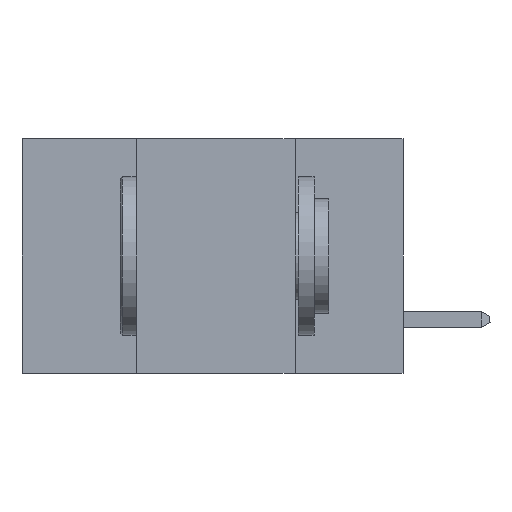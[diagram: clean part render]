
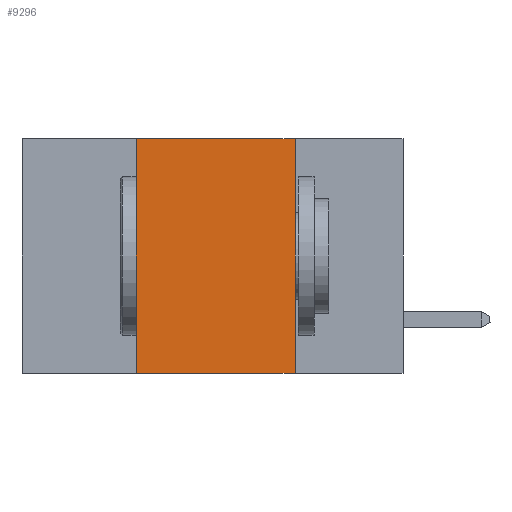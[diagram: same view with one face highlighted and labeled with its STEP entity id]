
A CAD part, left-side view. The second image highlights one B-rep face of the part: STEP entity #9296.
In plain terms, the highlighted planar face has unit normal (-1, 0, 0).
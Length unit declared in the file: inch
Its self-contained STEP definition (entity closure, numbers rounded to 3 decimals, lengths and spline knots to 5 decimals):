
#333 = CARTESIAN_POINT ( 'NONE',  ( 0., 0.17, 0. ) ) ;
#1075 = DIRECTION ( 'NONE',  ( 0., 0., -1. ) ) ;
#1240 = VECTOR ( 'NONE', #12766, 39.37008 ) ;
#1314 = CARTESIAN_POINT ( 'NONE',  ( 0., 0.17, -0.37 ) ) ;
#1398 = CARTESIAN_POINT ( 'NONE',  ( 0., 0.42, -0.37 ) ) ;
#2031 = CARTESIAN_POINT ( 'NONE',  ( 0., 0.42, 0. ) ) ;
#2140 = CARTESIAN_POINT ( 'NONE',  ( 0., 0.17, 0. ) ) ;
#2587 = EDGE_CURVE ( 'NONE', #10506, #12353, #2993, .T. ) ;
#2993 = LINE ( 'NONE', #2140, #11183 ) ;
#3273 = VECTOR ( 'NONE', #11204, 39.37008 ) ;
#3371 = CARTESIAN_POINT ( 'NONE',  ( 0., 0.6, 0. ) ) ;
#4138 = VECTOR ( 'NONE', #11100, 39.37008 ) ;
#4147 = EDGE_CURVE ( 'NONE', #7590, #10506, #11993, .T. ) ;
#4740 = AXIS2_PLACEMENT_3D ( 'NONE', #3371, #10365, #7177 ) ;
#4806 = PLANE ( 'NONE',  #4740 ) ;
#4901 = EDGE_LOOP ( 'NONE', ( #7902, #10625, #11329, #6994 ) ) ;
#6089 = LINE ( 'NONE', #8992, #3273 ) ;
#6994 = ORIENTED_EDGE ( 'NONE', *, *, #11892, .T. ) ;
#7177 = DIRECTION ( 'NONE',  ( 0., 0., -1. ) ) ;
#7590 = VERTEX_POINT ( 'NONE', #2031 ) ;
#7795 = EDGE_CURVE ( 'NONE', #11378, #7590, #12609, .T. ) ;
#7902 = ORIENTED_EDGE ( 'NONE', *, *, #2587, .F. ) ;
#8992 = CARTESIAN_POINT ( 'NONE',  ( 0., 0.6, -0.37 ) ) ;
#9296 = ADVANCED_FACE ( 'NONE', ( #10051 ), #4806, .F. ) ;
#9665 = CARTESIAN_POINT ( 'NONE',  ( 0., 0.42, 0. ) ) ;
#10051 = FACE_OUTER_BOUND ( 'NONE', #4901, .T. ) ;
#10265 = CARTESIAN_POINT ( 'NONE',  ( 0., 0.6, 0. ) ) ;
#10365 = DIRECTION ( 'NONE',  ( 1., 0., 0. ) ) ;
#10506 = VERTEX_POINT ( 'NONE', #333 ) ;
#10625 = ORIENTED_EDGE ( 'NONE', *, *, #4147, .F. ) ;
#11100 = DIRECTION ( 'NONE',  ( 0., -1., 0. ) ) ;
#11183 = VECTOR ( 'NONE', #1075, 39.37008 ) ;
#11204 = DIRECTION ( 'NONE',  ( 0., -1., 0. ) ) ;
#11329 = ORIENTED_EDGE ( 'NONE', *, *, #7795, .F. ) ;
#11378 = VERTEX_POINT ( 'NONE', #1398 ) ;
#11892 = EDGE_CURVE ( 'NONE', #11378, #12353, #6089, .T. ) ;
#11993 = LINE ( 'NONE', #10265, #4138 ) ;
#12353 = VERTEX_POINT ( 'NONE', #1314 ) ;
#12609 = LINE ( 'NONE', #9665, #1240 ) ;
#12766 = DIRECTION ( 'NONE',  ( 0., 0., 1. ) ) ;
